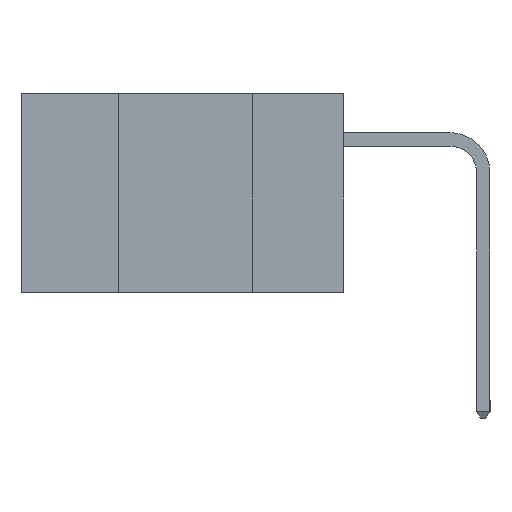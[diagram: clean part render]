
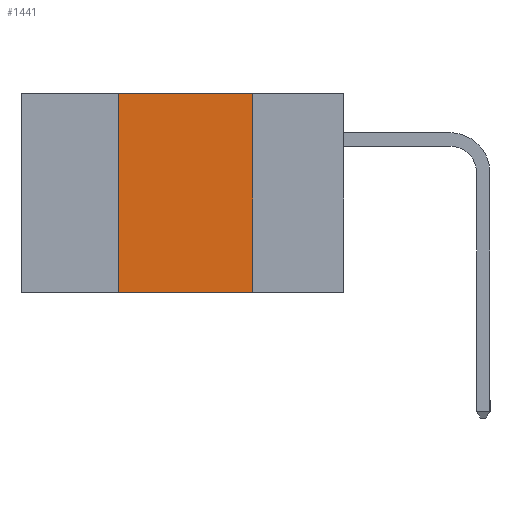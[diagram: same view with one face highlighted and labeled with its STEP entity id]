
A CAD part, left-side view. The second image highlights one B-rep face of the part: STEP entity #1441.
In plain terms, the highlighted planar face has unit normal (-1, 0, 0).
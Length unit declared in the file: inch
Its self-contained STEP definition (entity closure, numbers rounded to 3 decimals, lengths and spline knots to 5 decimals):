
#200 = LINE ( 'NONE', #3532, #2341 ) ;
#464 = DIRECTION ( 'NONE',  ( 0., -1., 0. ) ) ;
#737 = EDGE_CURVE ( 'NONE', #5735, #6733, #7587, .T. ) ;
#815 = EDGE_LOOP ( 'NONE', ( #4662, #2441, #4904, #9010 ) ) ;
#1075 = AXIS2_PLACEMENT_3D ( 'NONE', #9327, #10000, #4406 ) ;
#1200 = CARTESIAN_POINT ( 'NONE',  ( 0., 0.42, 0. ) ) ;
#1441 = ADVANCED_FACE ( 'NONE', ( #8331 ), #8048, .F. ) ;
#1485 = CARTESIAN_POINT ( 'NONE',  ( 0., 0.42, -0.37 ) ) ;
#2341 = VECTOR ( 'NONE', #7220, 39.37008 ) ;
#2441 = ORIENTED_EDGE ( 'NONE', *, *, #737, .F. ) ;
#2558 = EDGE_CURVE ( 'NONE', #3600, #3482, #9791, .T. ) ;
#2789 = VECTOR ( 'NONE', #8401, 39.37008 ) ;
#3482 = VERTEX_POINT ( 'NONE', #5815 ) ;
#3532 = CARTESIAN_POINT ( 'NONE',  ( 0., 0.17, -0.37 ) ) ;
#3600 = VERTEX_POINT ( 'NONE', #6723 ) ;
#4406 = DIRECTION ( 'NONE',  ( 0., 0., -1. ) ) ;
#4662 = ORIENTED_EDGE ( 'NONE', *, *, #9824, .F. ) ;
#4844 = LINE ( 'NONE', #1485, #2789 ) ;
#4904 = ORIENTED_EDGE ( 'NONE', *, *, #9523, .F. ) ;
#5735 = VERTEX_POINT ( 'NONE', #1200 ) ;
#5815 = CARTESIAN_POINT ( 'NONE',  ( 0., 0.17, -0.37 ) ) ;
#6181 = CARTESIAN_POINT ( 'NONE',  ( 0., 0.17, 0. ) ) ;
#6723 = CARTESIAN_POINT ( 'NONE',  ( 0., 0.42, -0.37 ) ) ;
#6733 = VERTEX_POINT ( 'NONE', #6181 ) ;
#7220 = DIRECTION ( 'NONE',  ( 0., 0., -1. ) ) ;
#7587 = LINE ( 'NONE', #8923, #8025 ) ;
#7715 = VECTOR ( 'NONE', #8701, 39.37008 ) ;
#8025 = VECTOR ( 'NONE', #464, 39.37008 ) ;
#8048 = PLANE ( 'NONE',  #1075 ) ;
#8331 = FACE_OUTER_BOUND ( 'NONE', #815, .T. ) ;
#8401 = DIRECTION ( 'NONE',  ( 0., 0., 1. ) ) ;
#8701 = DIRECTION ( 'NONE',  ( 0., -1., 0. ) ) ;
#8893 = CARTESIAN_POINT ( 'NONE',  ( 0., 0.6, -0.37 ) ) ;
#8923 = CARTESIAN_POINT ( 'NONE',  ( 0., 0.6, 0. ) ) ;
#9010 = ORIENTED_EDGE ( 'NONE', *, *, #2558, .T. ) ;
#9327 = CARTESIAN_POINT ( 'NONE',  ( 0., 0.6, 0. ) ) ;
#9523 = EDGE_CURVE ( 'NONE', #3600, #5735, #4844, .T. ) ;
#9791 = LINE ( 'NONE', #8893, #7715 ) ;
#9824 = EDGE_CURVE ( 'NONE', #6733, #3482, #200, .T. ) ;
#10000 = DIRECTION ( 'NONE',  ( 1., 0., 0. ) ) ;
